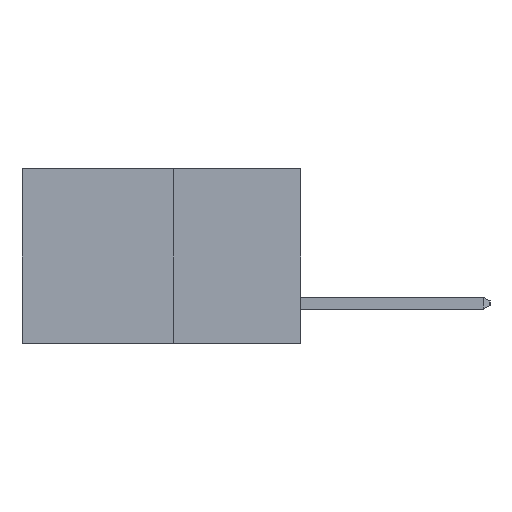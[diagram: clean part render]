
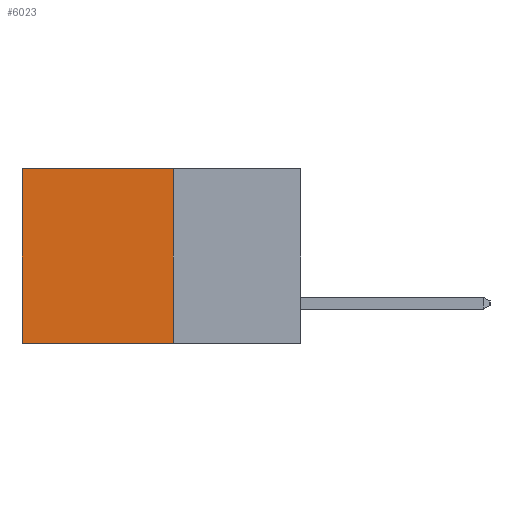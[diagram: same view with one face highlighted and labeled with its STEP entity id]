
A CAD part, left-side view. The second image highlights one B-rep face of the part: STEP entity #6023.
In plain terms, the highlighted planar face has unit normal (-1, 0, 0).
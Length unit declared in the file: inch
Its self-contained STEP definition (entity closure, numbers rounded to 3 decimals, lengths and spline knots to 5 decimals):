
#91 = EDGE_CURVE ( 'NONE', #7778, #9444, #976, .T. ) ;
#399 = ORIENTED_EDGE ( 'NONE', *, *, #7173, .F. ) ;
#485 = EDGE_CURVE ( 'NONE', #10729, #9444, #4431, .T. ) ;
#752 = DIRECTION ( 'NONE',  ( 0., 0., -1. ) ) ;
#775 = CARTESIAN_POINT ( 'NONE',  ( 0.277, 0.27, -0.37 ) ) ;
#976 = LINE ( 'NONE', #994, #9897 ) ;
#994 = CARTESIAN_POINT ( 'NONE',  ( 0.277, 0.59, -0.37 ) ) ;
#1540 = DIRECTION ( 'NONE',  ( 0., 1., 0. ) ) ;
#1707 = EDGE_LOOP ( 'NONE', ( #6084, #2743, #399, #1771 ) ) ;
#1771 = ORIENTED_EDGE ( 'NONE', *, *, #9938, .T. ) ;
#1965 = VECTOR ( 'NONE', #1540, 39.37008 ) ;
#2235 = CARTESIAN_POINT ( 'NONE',  ( 0.277, 0.27, -0.37 ) ) ;
#2290 = VERTEX_POINT ( 'NONE', #3983 ) ;
#2357 = FACE_OUTER_BOUND ( 'NONE', #1707, .T. ) ;
#2459 = CARTESIAN_POINT ( 'NONE',  ( 0.277, 0.59, -0.37 ) ) ;
#2743 = ORIENTED_EDGE ( 'NONE', *, *, #485, .F. ) ;
#2856 = CARTESIAN_POINT ( 'NONE',  ( 0.277, 0.59, 0. ) ) ;
#3655 = VECTOR ( 'NONE', #8354, 39.37008 ) ;
#3983 = CARTESIAN_POINT ( 'NONE',  ( 0.277, 0.27, 0. ) ) ;
#4363 = PLANE ( 'NONE',  #5439 ) ;
#4394 = CARTESIAN_POINT ( 'NONE',  ( 0.277, 0.27, -0.37 ) ) ;
#4431 = LINE ( 'NONE', #2235, #10783 ) ;
#4957 = CARTESIAN_POINT ( 'NONE',  ( 0.277, 0.27, -0.37 ) ) ;
#5245 = DIRECTION ( 'NONE',  ( 0., 0., -1. ) ) ;
#5439 = AXIS2_PLACEMENT_3D ( 'NONE', #4394, #10200, #5245 ) ;
#5855 = LINE ( 'NONE', #775, #3655 ) ;
#6023 = ADVANCED_FACE ( 'NONE', ( #2357 ), #4363, .F. ) ;
#6084 = ORIENTED_EDGE ( 'NONE', *, *, #91, .T. ) ;
#6429 = LINE ( 'NONE', #8216, #1965 ) ;
#6628 = DIRECTION ( 'NONE',  ( 0., 1., 0. ) ) ;
#7173 = EDGE_CURVE ( 'NONE', #2290, #10729, #5855, .T. ) ;
#7778 = VERTEX_POINT ( 'NONE', #2856 ) ;
#8216 = CARTESIAN_POINT ( 'NONE',  ( 0.277, 0.27, 0. ) ) ;
#8354 = DIRECTION ( 'NONE',  ( 0., 0., -1. ) ) ;
#9444 = VERTEX_POINT ( 'NONE', #2459 ) ;
#9897 = VECTOR ( 'NONE', #752, 39.37008 ) ;
#9938 = EDGE_CURVE ( 'NONE', #2290, #7778, #6429, .T. ) ;
#10200 = DIRECTION ( 'NONE',  ( 1., 0., 0. ) ) ;
#10729 = VERTEX_POINT ( 'NONE', #4957 ) ;
#10783 = VECTOR ( 'NONE', #6628, 39.37008 ) ;
